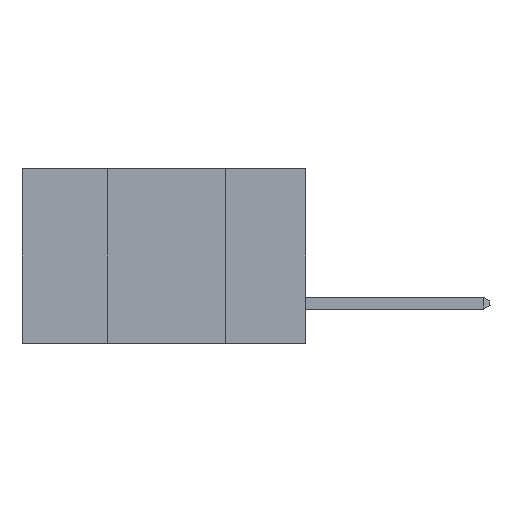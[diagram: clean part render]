
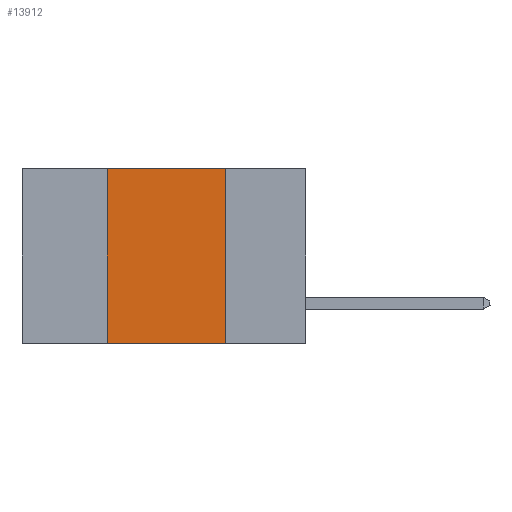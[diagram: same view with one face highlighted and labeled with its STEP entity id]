
A CAD part, left-side view. The second image highlights one B-rep face of the part: STEP entity #13912.
In plain terms, the highlighted planar face has unit normal (-1, 0, 0).
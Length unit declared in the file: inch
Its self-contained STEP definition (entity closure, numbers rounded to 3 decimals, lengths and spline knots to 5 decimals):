
#512 = ORIENTED_EDGE ( 'NONE', *, *, #13942, .F. ) ;
#894 = FACE_OUTER_BOUND ( 'NONE', #12296, .T. ) ;
#1367 = VERTEX_POINT ( 'NONE', #12432 ) ;
#1578 = VECTOR ( 'NONE', #11227, 39.37008 ) ;
#2251 = EDGE_CURVE ( 'NONE', #12630, #5233, #2504, .T. ) ;
#2504 = LINE ( 'NONE', #11618, #12391 ) ;
#2651 = EDGE_CURVE ( 'NONE', #12630, #1367, #4646, .T. ) ;
#3702 = VECTOR ( 'NONE', #10252, 39.37008 ) ;
#3991 = AXIS2_PLACEMENT_3D ( 'NONE', #14579, #12285, #5407 ) ;
#4090 = ORIENTED_EDGE ( 'NONE', *, *, #2251, .F. ) ;
#4161 = ORIENTED_EDGE ( 'NONE', *, *, #2651, .T. ) ;
#4646 = LINE ( 'NONE', #6546, #1578 ) ;
#4732 = DIRECTION ( 'NONE',  ( 0., 0., 1. ) ) ;
#5233 = VERTEX_POINT ( 'NONE', #12370 ) ;
#5407 = DIRECTION ( 'NONE',  ( 0., 0., -1. ) ) ;
#6546 = CARTESIAN_POINT ( 'NONE',  ( 0., 0.6, -0.37 ) ) ;
#7195 = VECTOR ( 'NONE', #13994, 39.37008 ) ;
#7667 = EDGE_CURVE ( 'NONE', #5233, #13432, #14163, .T. ) ;
#7882 = CARTESIAN_POINT ( 'NONE',  ( 0., 0.42, -0.37 ) ) ;
#8498 = CARTESIAN_POINT ( 'NONE',  ( 0., 0.17, 0. ) ) ;
#10252 = DIRECTION ( 'NONE',  ( 0., -1., 0. ) ) ;
#10278 = LINE ( 'NONE', #13237, #7195 ) ;
#11227 = DIRECTION ( 'NONE',  ( 0., -1., 0. ) ) ;
#11618 = CARTESIAN_POINT ( 'NONE',  ( 0., 0.42, -0.37 ) ) ;
#12285 = DIRECTION ( 'NONE',  ( 1., 0., 0. ) ) ;
#12296 = EDGE_LOOP ( 'NONE', ( #512, #14002, #4090, #4161 ) ) ;
#12370 = CARTESIAN_POINT ( 'NONE',  ( 0., 0.42, 0. ) ) ;
#12391 = VECTOR ( 'NONE', #4732, 39.37008 ) ;
#12432 = CARTESIAN_POINT ( 'NONE',  ( 0., 0.17, -0.37 ) ) ;
#12495 = CARTESIAN_POINT ( 'NONE',  ( 0., 0.6, 0. ) ) ;
#12630 = VERTEX_POINT ( 'NONE', #7882 ) ;
#13237 = CARTESIAN_POINT ( 'NONE',  ( 0., 0.17, -0.37 ) ) ;
#13297 = PLANE ( 'NONE',  #3991 ) ;
#13432 = VERTEX_POINT ( 'NONE', #8498 ) ;
#13912 = ADVANCED_FACE ( 'NONE', ( #894 ), #13297, .F. ) ;
#13942 = EDGE_CURVE ( 'NONE', #13432, #1367, #10278, .T. ) ;
#13994 = DIRECTION ( 'NONE',  ( 0., 0., -1. ) ) ;
#14002 = ORIENTED_EDGE ( 'NONE', *, *, #7667, .F. ) ;
#14163 = LINE ( 'NONE', #12495, #3702 ) ;
#14579 = CARTESIAN_POINT ( 'NONE',  ( 0., 0.6, 0. ) ) ;
